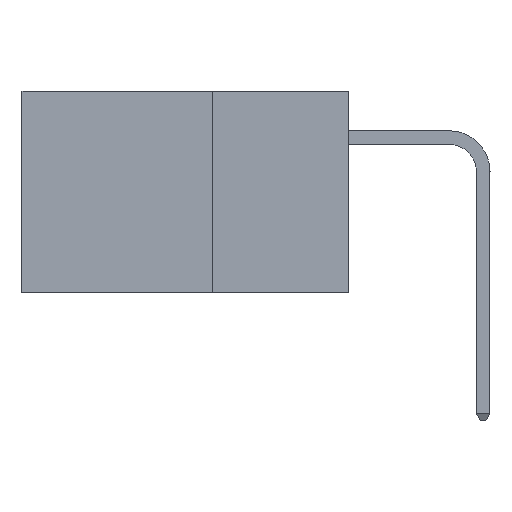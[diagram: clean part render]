
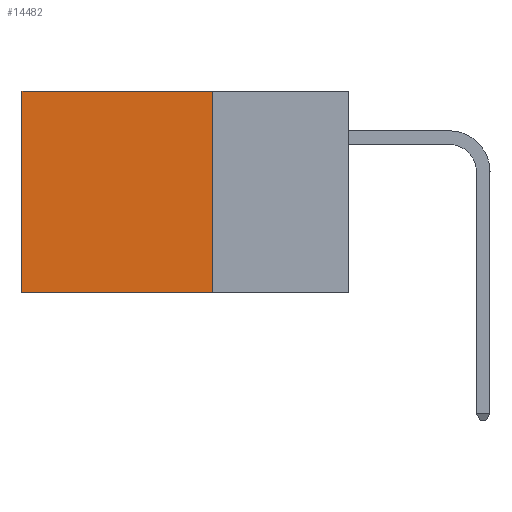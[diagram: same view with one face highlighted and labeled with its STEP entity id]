
A CAD part, left-side view. The second image highlights one B-rep face of the part: STEP entity #14482.
In plain terms, the highlighted planar face has unit normal (-1, 0, 0).
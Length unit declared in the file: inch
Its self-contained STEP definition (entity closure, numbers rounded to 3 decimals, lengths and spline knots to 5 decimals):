
#280 = VECTOR ( 'NONE', #682, 39.37008 ) ;
#294 = CARTESIAN_POINT ( 'NONE',  ( 0.2875, 0.25, 0. ) ) ;
#334 = CARTESIAN_POINT ( 'NONE',  ( 0.2875, 0.25, 0. ) ) ;
#636 = EDGE_CURVE ( 'NONE', #15272, #13948, #667, .T. ) ;
#667 = LINE ( 'NONE', #294, #15042 ) ;
#682 = DIRECTION ( 'NONE',  ( 0., 0., -1. ) ) ;
#969 = ORIENTED_EDGE ( 'NONE', *, *, #7610, .F. ) ;
#1138 = DIRECTION ( 'NONE',  ( 0., 0., -1. ) ) ;
#1477 = CARTESIAN_POINT ( 'NONE',  ( 0.2875, 0.25, -0.37 ) ) ;
#2423 = CARTESIAN_POINT ( 'NONE',  ( 0.2875, 0.25, 0. ) ) ;
#2710 = VERTEX_POINT ( 'NONE', #15151 ) ;
#3928 = ORIENTED_EDGE ( 'NONE', *, *, #12703, .T. ) ;
#4246 = ORIENTED_EDGE ( 'NONE', *, *, #14090, .F. ) ;
#5444 = DIRECTION ( 'NONE',  ( 0., 0., -1. ) ) ;
#5638 = AXIS2_PLACEMENT_3D ( 'NONE', #2423, #9538, #1138 ) ;
#6775 = CARTESIAN_POINT ( 'NONE',  ( 0.2875, 0.6, 0. ) ) ;
#7610 = EDGE_CURVE ( 'NONE', #15272, #13555, #15096, .T. ) ;
#7626 = ORIENTED_EDGE ( 'NONE', *, *, #636, .T. ) ;
#8312 = LINE ( 'NONE', #6775, #16631 ) ;
#9356 = DIRECTION ( 'NONE',  ( 0., 1., 0. ) ) ;
#9380 = EDGE_LOOP ( 'NONE', ( #3928, #4246, #969, #7626 ) ) ;
#9538 = DIRECTION ( 'NONE',  ( 1., 0., 0. ) ) ;
#9577 = DIRECTION ( 'NONE',  ( 0., 1., 0. ) ) ;
#9728 = CARTESIAN_POINT ( 'NONE',  ( 0.2875, 0.25, -0.37 ) ) ;
#11956 = CARTESIAN_POINT ( 'NONE',  ( 0.2875, 0.25, 0. ) ) ;
#12326 = CARTESIAN_POINT ( 'NONE',  ( 0.2875, 0.6, 0. ) ) ;
#12703 = EDGE_CURVE ( 'NONE', #13948, #2710, #8312, .T. ) ;
#13555 = VERTEX_POINT ( 'NONE', #9728 ) ;
#13675 = PLANE ( 'NONE',  #5638 ) ;
#13706 = LINE ( 'NONE', #1477, #16354 ) ;
#13910 = FACE_OUTER_BOUND ( 'NONE', #9380, .T. ) ;
#13948 = VERTEX_POINT ( 'NONE', #12326 ) ;
#14090 = EDGE_CURVE ( 'NONE', #13555, #2710, #13706, .T. ) ;
#14482 = ADVANCED_FACE ( 'NONE', ( #13910 ), #13675, .F. ) ;
#15042 = VECTOR ( 'NONE', #9356, 39.37008 ) ;
#15096 = LINE ( 'NONE', #11956, #280 ) ;
#15151 = CARTESIAN_POINT ( 'NONE',  ( 0.2875, 0.6, -0.37 ) ) ;
#15272 = VERTEX_POINT ( 'NONE', #334 ) ;
#16354 = VECTOR ( 'NONE', #9577, 39.37008 ) ;
#16631 = VECTOR ( 'NONE', #5444, 39.37008 ) ;
